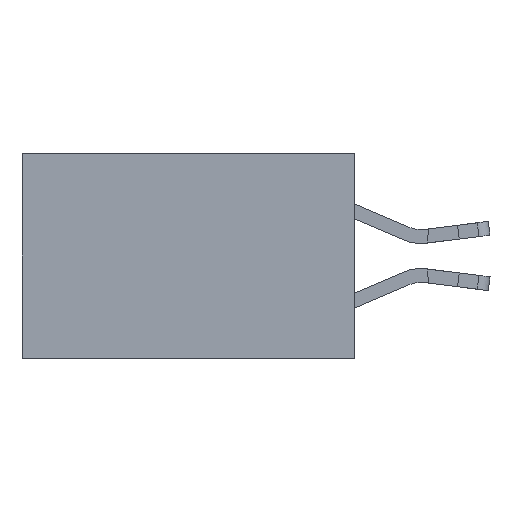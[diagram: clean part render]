
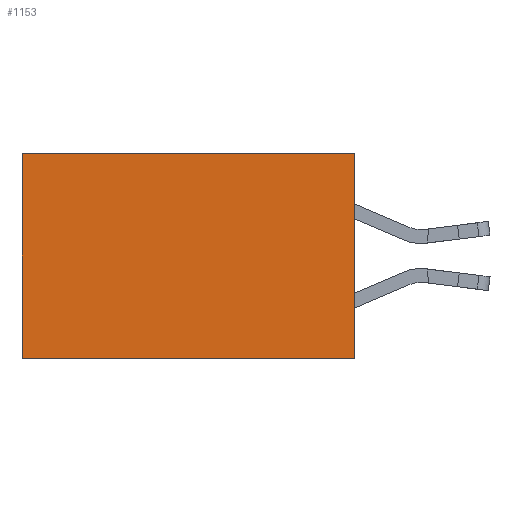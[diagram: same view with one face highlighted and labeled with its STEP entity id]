
A CAD part, left-side view. The second image highlights one B-rep face of the part: STEP entity #1153.
In plain terms, the highlighted planar face has unit normal (-1, 0, 0).
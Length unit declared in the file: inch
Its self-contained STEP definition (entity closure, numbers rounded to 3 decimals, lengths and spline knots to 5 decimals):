
#1153 = ADVANCED_FACE ( 'NONE', ( #3473 ), #4564, .F. ) ;
#1448 = LINE ( 'NONE', #8576, #7223 ) ;
#2238 = EDGE_CURVE ( 'NONE', #18126, #18898, #5105, .T. ) ;
#3473 = FACE_OUTER_BOUND ( 'NONE', #9242, .T. ) ;
#3502 = CARTESIAN_POINT ( 'NONE',  ( 0.298, 0., -0.37 ) ) ;
#4564 = PLANE ( 'NONE',  #18024 ) ;
#5105 = LINE ( 'NONE', #17451, #17979 ) ;
#5510 = ORIENTED_EDGE ( 'NONE', *, *, #10302, .F. ) ;
#6219 = VERTEX_POINT ( 'NONE', #9649 ) ;
#7121 = LINE ( 'NONE', #3502, #17565 ) ;
#7223 = VECTOR ( 'NONE', #16052, 39.37008 ) ;
#7436 = CARTESIAN_POINT ( 'NONE',  ( 0.298, 0., 0. ) ) ;
#7568 = DIRECTION ( 'NONE',  ( 0., 0., -1. ) ) ;
#8113 = LINE ( 'NONE', #13085, #9751 ) ;
#8311 = CARTESIAN_POINT ( 'NONE',  ( 0.298, 0., -0.37 ) ) ;
#8576 = CARTESIAN_POINT ( 'NONE',  ( 0.298, 0.6, 0. ) ) ;
#9242 = EDGE_LOOP ( 'NONE', ( #13891, #5510, #15270, #12986 ) ) ;
#9649 = CARTESIAN_POINT ( 'NONE',  ( 0.298, 0.6, 0. ) ) ;
#9651 = DIRECTION ( 'NONE',  ( 0., 1., 0. ) ) ;
#9751 = VECTOR ( 'NONE', #11513, 39.37008 ) ;
#10302 = EDGE_CURVE ( 'NONE', #18898, #11537, #7121, .T. ) ;
#11513 = DIRECTION ( 'NONE',  ( 0., 1., 0. ) ) ;
#11537 = VERTEX_POINT ( 'NONE', #19570 ) ;
#12986 = ORIENTED_EDGE ( 'NONE', *, *, #13125, .T. ) ;
#13085 = CARTESIAN_POINT ( 'NONE',  ( 0.298, 0., 0. ) ) ;
#13125 = EDGE_CURVE ( 'NONE', #18126, #6219, #8113, .T. ) ;
#13891 = ORIENTED_EDGE ( 'NONE', *, *, #18977, .T. ) ;
#15270 = ORIENTED_EDGE ( 'NONE', *, *, #2238, .F. ) ;
#15319 = DIRECTION ( 'NONE',  ( 1., 0., 0. ) ) ;
#16052 = DIRECTION ( 'NONE',  ( 0., 0., -1. ) ) ;
#16851 = DIRECTION ( 'NONE',  ( 0., 0., -1. ) ) ;
#17451 = CARTESIAN_POINT ( 'NONE',  ( 0.298, 0., 0. ) ) ;
#17565 = VECTOR ( 'NONE', #9651, 39.37008 ) ;
#17979 = VECTOR ( 'NONE', #7568, 39.37008 ) ;
#18024 = AXIS2_PLACEMENT_3D ( 'NONE', #18319, #15319, #16851 ) ;
#18126 = VERTEX_POINT ( 'NONE', #7436 ) ;
#18319 = CARTESIAN_POINT ( 'NONE',  ( 0.298, 0., 0. ) ) ;
#18898 = VERTEX_POINT ( 'NONE', #8311 ) ;
#18977 = EDGE_CURVE ( 'NONE', #6219, #11537, #1448, .T. ) ;
#19570 = CARTESIAN_POINT ( 'NONE',  ( 0.298, 0.6, -0.37 ) ) ;
